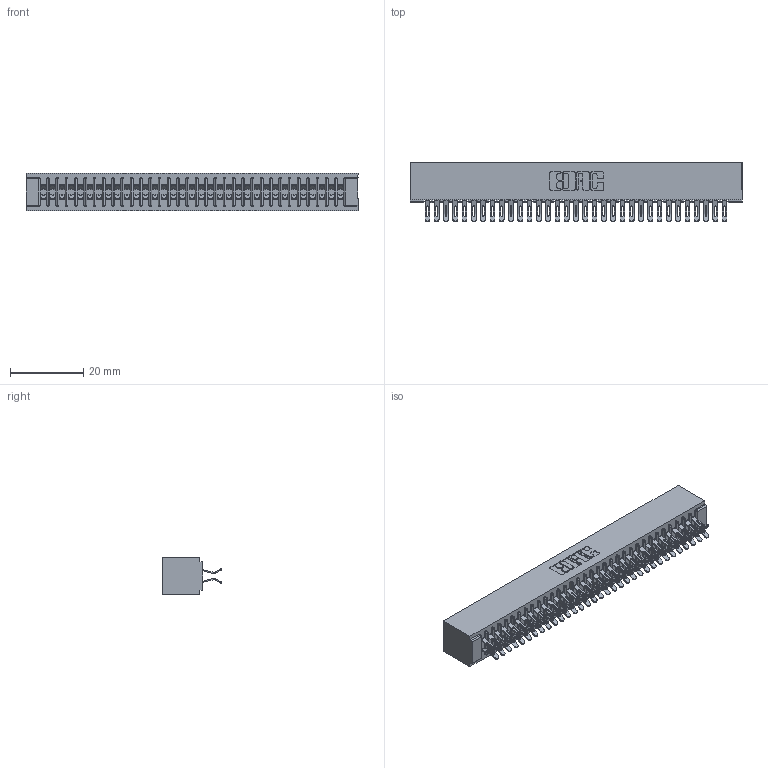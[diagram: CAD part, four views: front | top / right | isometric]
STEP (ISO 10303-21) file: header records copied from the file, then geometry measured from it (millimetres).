
FILE_DESCRIPTION (( 'STEP AP203' ), '1' );
FILE_NAME ('391-066-555-201.STEP', '2018-08-09T13:32:29', ( '' ), ( '' ), 'SwSTEP 2.0', 'SolidWorks 2016', '' );
FILE_SCHEMA (( 'CONFIG_CONTROL_DESIGN' ));
Length unit declared in the file: inch
Products named in the file (3): 341-292-001_341-292-155; 391-066-555-201; 341 Part_No Mounting Lugs
Assembly tree (67 placements, depth 2):
  391-066-555-201
    341 Part_No Mounting Lugs
    341-292-001_341-292-155  x66
Bounding box: 90.81 x 16.31 x 10.16 mm (x, y, z)
Volume: 7017.3 mm3; surface area: 13373.3 mm2
Topology: 67 solids, 67 shells, 5256 faces, 15703 edges, 10222 vertices
Faces by surface type: plane 2836, cylinder 2288, sphere 68, torus 64
Entity records: 41328 total; most frequent: CARTESIAN_POINT 6885, ORIENTED_EDGE 6830, DIRECTION 6677, EDGE_CURVE 3415, VECTOR 2737, LINE 2737, VERTEX_POINT 2162, AXIS2_PLACEMENT_3D 1970
